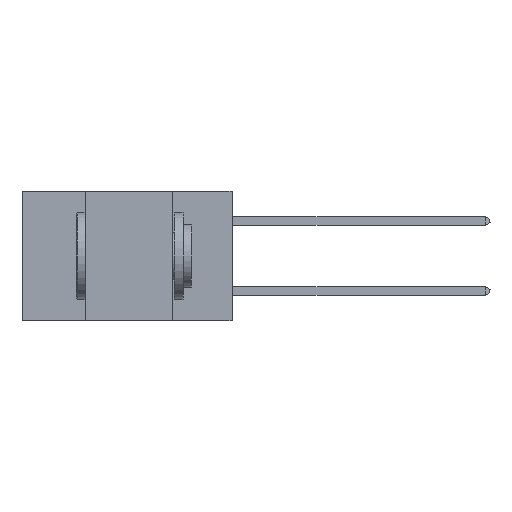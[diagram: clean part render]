
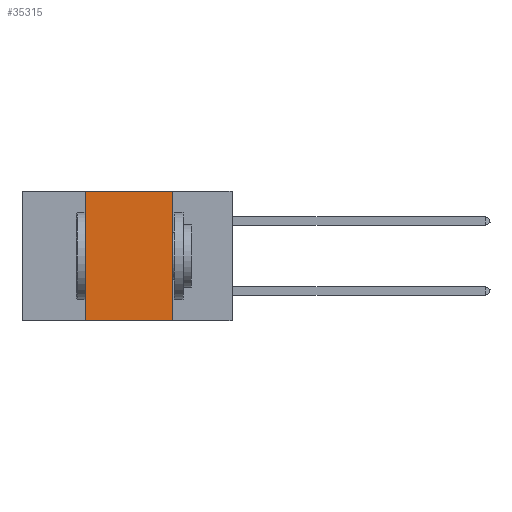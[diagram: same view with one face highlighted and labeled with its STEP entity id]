
A CAD part, left-side view. The second image highlights one B-rep face of the part: STEP entity #35315.
In plain terms, the highlighted planar face has unit normal (-1, 0, 0).
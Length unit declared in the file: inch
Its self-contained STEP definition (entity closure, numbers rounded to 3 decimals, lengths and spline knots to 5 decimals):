
#2932 = CARTESIAN_POINT ( 'NONE',  ( 0., 0.42, 0. ) ) ;
#8066 = DIRECTION ( 'NONE',  ( 0., -1., 0. ) ) ;
#8895 = EDGE_CURVE ( 'NONE', #29639, #17423, #37314, .T. ) ;
#9701 = PLANE ( 'NONE',  #27812 ) ;
#10260 = EDGE_CURVE ( 'NONE', #25288, #35764, #34057, .T. ) ;
#12129 = ORIENTED_EDGE ( 'NONE', *, *, #8895, .F. ) ;
#12732 = CARTESIAN_POINT ( 'NONE',  ( 0., 0.17, 0. ) ) ;
#12769 = CARTESIAN_POINT ( 'NONE',  ( 0., 0.6, 0. ) ) ;
#13070 = LINE ( 'NONE', #31821, #28872 ) ;
#13430 = EDGE_LOOP ( 'NONE', ( #19123, #34938, #12129, #37677 ) ) ;
#13665 = VECTOR ( 'NONE', #24357, 39.37008 ) ;
#15753 = DIRECTION ( 'NONE',  ( 1., 0., 0. ) ) ;
#16270 = CARTESIAN_POINT ( 'NONE',  ( 0., 0.6, -0.37 ) ) ;
#17423 = VERTEX_POINT ( 'NONE', #2932 ) ;
#18241 = VECTOR ( 'NONE', #33531, 39.37008 ) ;
#19123 = ORIENTED_EDGE ( 'NONE', *, *, #10260, .F. ) ;
#20402 = EDGE_CURVE ( 'NONE', #29639, #35764, #28161, .T. ) ;
#20501 = CARTESIAN_POINT ( 'NONE',  ( 0., 0.17, -0.37 ) ) ;
#21196 = VECTOR ( 'NONE', #28078, 39.37008 ) ;
#21395 = CARTESIAN_POINT ( 'NONE',  ( 0., 0.42, 0. ) ) ;
#24357 = DIRECTION ( 'NONE',  ( 0., 0., 1. ) ) ;
#25288 = VERTEX_POINT ( 'NONE', #31176 ) ;
#27812 = AXIS2_PLACEMENT_3D ( 'NONE', #12769, #15753, #36517 ) ;
#28078 = DIRECTION ( 'NONE',  ( 0., -1., 0. ) ) ;
#28161 = LINE ( 'NONE', #16270, #21196 ) ;
#28872 = VECTOR ( 'NONE', #8066, 39.37008 ) ;
#29639 = VERTEX_POINT ( 'NONE', #34934 ) ;
#31176 = CARTESIAN_POINT ( 'NONE',  ( 0., 0.17, 0. ) ) ;
#31821 = CARTESIAN_POINT ( 'NONE',  ( 0., 0.6, 0. ) ) ;
#32669 = EDGE_CURVE ( 'NONE', #17423, #25288, #13070, .T. ) ;
#33531 = DIRECTION ( 'NONE',  ( 0., 0., -1. ) ) ;
#34057 = LINE ( 'NONE', #12732, #18241 ) ;
#34934 = CARTESIAN_POINT ( 'NONE',  ( 0., 0.42, -0.37 ) ) ;
#34938 = ORIENTED_EDGE ( 'NONE', *, *, #32669, .F. ) ;
#35315 = ADVANCED_FACE ( 'NONE', ( #36158 ), #9701, .F. ) ;
#35764 = VERTEX_POINT ( 'NONE', #20501 ) ;
#36158 = FACE_OUTER_BOUND ( 'NONE', #13430, .T. ) ;
#36517 = DIRECTION ( 'NONE',  ( 0., 0., -1. ) ) ;
#37314 = LINE ( 'NONE', #21395, #13665 ) ;
#37677 = ORIENTED_EDGE ( 'NONE', *, *, #20402, .T. ) ;
